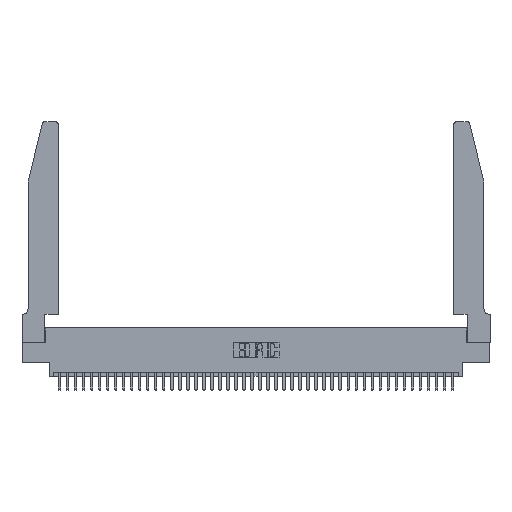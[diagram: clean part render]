
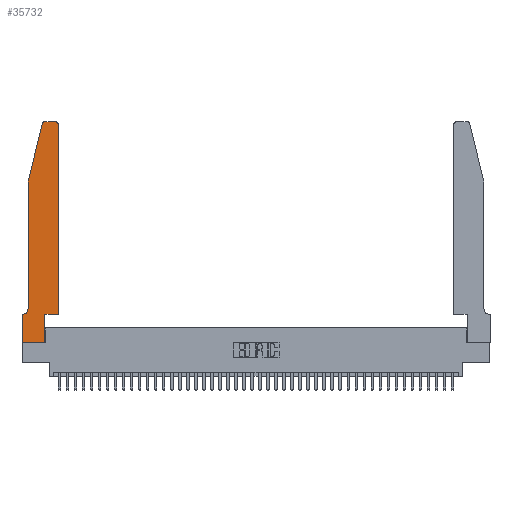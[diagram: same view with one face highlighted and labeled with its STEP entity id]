
A CAD part, top view. The second image highlights one B-rep face of the part: STEP entity #35732.
In plain terms, the highlighted planar face has unit normal (0, 0, 1).
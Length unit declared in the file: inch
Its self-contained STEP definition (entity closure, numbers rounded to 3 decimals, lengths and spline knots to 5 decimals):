
#336 = VECTOR ( 'NONE', #29955, 39.37008 ) ;
#1230 = LINE ( 'NONE', #37731, #14378 ) ;
#2190 = DIRECTION ( 'NONE',  ( -1., 0., 0. ) ) ;
#2556 = ORIENTED_EDGE ( 'NONE', *, *, #33595, .T. ) ;
#2666 = CARTESIAN_POINT ( 'NONE',  ( 0.0755, 2., 0.37 ) ) ;
#3342 = CARTESIAN_POINT ( 'NONE',  ( 0.284, 2.72, 0.37 ) ) ;
#3550 = CARTESIAN_POINT ( 'NONE',  ( 0.0755, 0.35, 0.37 ) ) ;
#4977 = CARTESIAN_POINT ( 'NONE',  ( 0., 0.35, 0.37 ) ) ;
#5134 = DIRECTION ( 'NONE',  ( 0., 0., -1. ) ) ;
#5368 = VERTEX_POINT ( 'NONE', #40160 ) ;
#6055 = ORIENTED_EDGE ( 'NONE', *, *, #36726, .T. ) ;
#6203 = ORIENTED_EDGE ( 'NONE', *, *, #42505, .T. ) ;
#6680 = CARTESIAN_POINT ( 'NONE',  ( 0.284, 2.75, 0.37 ) ) ;
#7223 = EDGE_CURVE ( 'NONE', #7454, #39705, #1230, .T. ) ;
#7278 = CARTESIAN_POINT ( 'NONE',  ( 0.2605, 2.75, 0.37 ) ) ;
#7454 = VERTEX_POINT ( 'NONE', #29679 ) ;
#7466 = ORIENTED_EDGE ( 'NONE', *, *, #35857, .T. ) ;
#7788 = CARTESIAN_POINT ( 'NONE',  ( 0.0055, 0.35, 0.37 ) ) ;
#8381 = VERTEX_POINT ( 'NONE', #22951 ) ;
#9489 = VECTOR ( 'NONE', #24501, 39.37008 ) ;
#9520 = LINE ( 'NONE', #40715, #29821 ) ;
#9593 = ORIENTED_EDGE ( 'NONE', *, *, #30074, .T. ) ;
#9636 = VERTEX_POINT ( 'NONE', #12139 ) ;
#10265 = CARTESIAN_POINT ( 'NONE',  ( 0.2865, 0., 0.37 ) ) ;
#10450 = CARTESIAN_POINT ( 'NONE',  ( 0.0755, 0.42, 0.37 ) ) ;
#10530 = CARTESIAN_POINT ( 'NONE',  ( 0., 0., 0.37 ) ) ;
#10775 = VERTEX_POINT ( 'NONE', #6680 ) ;
#11373 = DIRECTION ( 'NONE',  ( 1., 0., 0. ) ) ;
#11893 = CARTESIAN_POINT ( 'NONE',  ( 0.0055, 0.42, 0.37 ) ) ;
#12139 = CARTESIAN_POINT ( 'NONE',  ( 0.0755, 2., 0.37 ) ) ;
#12357 = CARTESIAN_POINT ( 'NONE',  ( 0.2865, 0.35, 0.37 ) ) ;
#12794 = DIRECTION ( 'NONE',  ( 0., -1., 0. ) ) ;
#13155 = EDGE_CURVE ( 'NONE', #32030, #7454, #18293, .T. ) ;
#14378 = VECTOR ( 'NONE', #18256, 39.37008 ) ;
#14573 = CARTESIAN_POINT ( 'NONE',  ( 0.4205, 2.75, 0.37 ) ) ;
#14711 = CIRCLE ( 'NONE', #25540, 0.03 ) ;
#14716 = VECTOR ( 'NONE', #23525, 39.37008 ) ;
#14782 = AXIS2_PLACEMENT_3D ( 'NONE', #11893, #5134, #2190 ) ;
#15351 = VERTEX_POINT ( 'NONE', #10265 ) ;
#16662 = ORIENTED_EDGE ( 'NONE', *, *, #7223, .T. ) ;
#17193 = DIRECTION ( 'NONE',  ( 1., 0., 0. ) ) ;
#17467 = EDGE_CURVE ( 'NONE', #15351, #31405, #25758, .T. ) ;
#17690 = CIRCLE ( 'NONE', #14782, 0.07 ) ;
#18112 = DIRECTION ( 'NONE',  ( 1., 0., 0. ) ) ;
#18153 = LINE ( 'NONE', #7278, #336 ) ;
#18256 = DIRECTION ( 'NONE',  ( 0., -1., 0. ) ) ;
#18293 = LINE ( 'NONE', #3550, #9489 ) ;
#18722 = FACE_OUTER_BOUND ( 'NONE', #29439, .T. ) ;
#18793 = EDGE_CURVE ( 'NONE', #10775, #40141, #14711, .T. ) ;
#18896 = VECTOR ( 'NONE', #12794, 39.37008 ) ;
#19986 = VECTOR ( 'NONE', #43172, 39.37008 ) ;
#20042 = CARTESIAN_POINT ( 'NONE',  ( 0., 0., 0.37 ) ) ;
#20621 = VECTOR ( 'NONE', #23672, 39.37008 ) ;
#21152 = PLANE ( 'NONE',  #34838 ) ;
#21215 = DIRECTION ( 'NONE',  ( 0., 0., 1. ) ) ;
#22038 = ORIENTED_EDGE ( 'NONE', *, *, #24585, .T. ) ;
#22951 = CARTESIAN_POINT ( 'NONE',  ( 0.4505, 0.35, 0.37 ) ) ;
#23110 = CARTESIAN_POINT ( 'NONE',  ( 0.4505, 0.35, 0.37 ) ) ;
#23525 = DIRECTION ( 'NONE',  ( 0., 1., 0. ) ) ;
#23672 = DIRECTION ( 'NONE',  ( 1., 0., 0. ) ) ;
#24298 = CARTESIAN_POINT ( 'NONE',  ( 0.2865, 0.35, 0.37 ) ) ;
#24501 = DIRECTION ( 'NONE',  ( -1., 0., 0. ) ) ;
#24545 = LINE ( 'NONE', #23110, #14716 ) ;
#24585 = EDGE_CURVE ( 'NONE', #40141, #9636, #9520, .T. ) ;
#25014 = EDGE_CURVE ( 'NONE', #8381, #5368, #24545, .T. ) ;
#25540 = AXIS2_PLACEMENT_3D ( 'NONE', #3342, #26710, #17193 ) ;
#25758 = LINE ( 'NONE', #12357, #19986 ) ;
#26287 = VECTOR ( 'NONE', #27793, 39.37008 ) ;
#26710 = DIRECTION ( 'NONE',  ( 0., 0., 1. ) ) ;
#26795 = LINE ( 'NONE', #27507, #26287 ) ;
#27507 = CARTESIAN_POINT ( 'NONE',  ( 0.4505, 0.35, 0.37 ) ) ;
#27793 = DIRECTION ( 'NONE',  ( 1., 0., 0. ) ) ;
#28028 = ORIENTED_EDGE ( 'NONE', *, *, #13155, .T. ) ;
#28153 = CARTESIAN_POINT ( 'NONE',  ( 0.25487, 2.72718, 0.37 ) ) ;
#29439 = EDGE_LOOP ( 'NONE', ( #6055, #36906, #22038, #41679, #7466, #28028, #16662, #2556, #40208, #9593, #37684, #6203 ) ) ;
#29679 = CARTESIAN_POINT ( 'NONE',  ( 0., 0.35, 0.37 ) ) ;
#29821 = VECTOR ( 'NONE', #34214, 39.37008 ) ;
#29955 = DIRECTION ( 'NONE',  ( -1., 0., 0. ) ) ;
#30027 = AXIS2_PLACEMENT_3D ( 'NONE', #37796, #21215, #11373 ) ;
#30074 = EDGE_CURVE ( 'NONE', #31405, #8381, #26795, .T. ) ;
#30706 = EDGE_CURVE ( 'NONE', #9636, #37941, #33525, .T. ) ;
#31405 = VERTEX_POINT ( 'NONE', #24298 ) ;
#32030 = VERTEX_POINT ( 'NONE', #7788 ) ;
#33525 = LINE ( 'NONE', #2666, #18896 ) ;
#33595 = EDGE_CURVE ( 'NONE', #39705, #15351, #37275, .T. ) ;
#33627 = CIRCLE ( 'NONE', #30027, 0.03 ) ;
#34214 = DIRECTION ( 'NONE',  ( -0.239, -0.971, 0. ) ) ;
#34838 = AXIS2_PLACEMENT_3D ( 'NONE', #4977, #35008, #18112 ) ;
#35008 = DIRECTION ( 'NONE',  ( 0., 0., 1. ) ) ;
#35190 = VERTEX_POINT ( 'NONE', #14573 ) ;
#35732 = ADVANCED_FACE ( 'NONE', ( #18722 ), #21152, .T. ) ;
#35857 = EDGE_CURVE ( 'NONE', #37941, #32030, #17690, .T. ) ;
#36726 = EDGE_CURVE ( 'NONE', #35190, #10775, #18153, .T. ) ;
#36906 = ORIENTED_EDGE ( 'NONE', *, *, #18793, .T. ) ;
#37275 = LINE ( 'NONE', #20042, #20621 ) ;
#37684 = ORIENTED_EDGE ( 'NONE', *, *, #25014, .T. ) ;
#37731 = CARTESIAN_POINT ( 'NONE',  ( 0., 0., 0.37 ) ) ;
#37796 = CARTESIAN_POINT ( 'NONE',  ( 0.4205, 2.72, 0.37 ) ) ;
#37941 = VERTEX_POINT ( 'NONE', #10450 ) ;
#39705 = VERTEX_POINT ( 'NONE', #10530 ) ;
#40141 = VERTEX_POINT ( 'NONE', #28153 ) ;
#40160 = CARTESIAN_POINT ( 'NONE',  ( 0.4505, 2.72, 0.37 ) ) ;
#40208 = ORIENTED_EDGE ( 'NONE', *, *, #17467, .T. ) ;
#40715 = CARTESIAN_POINT ( 'NONE',  ( 0.0755, 2., 0.37 ) ) ;
#41679 = ORIENTED_EDGE ( 'NONE', *, *, #30706, .T. ) ;
#42505 = EDGE_CURVE ( 'NONE', #5368, #35190, #33627, .T. ) ;
#43172 = DIRECTION ( 'NONE',  ( 0., 1., 0. ) ) ;
